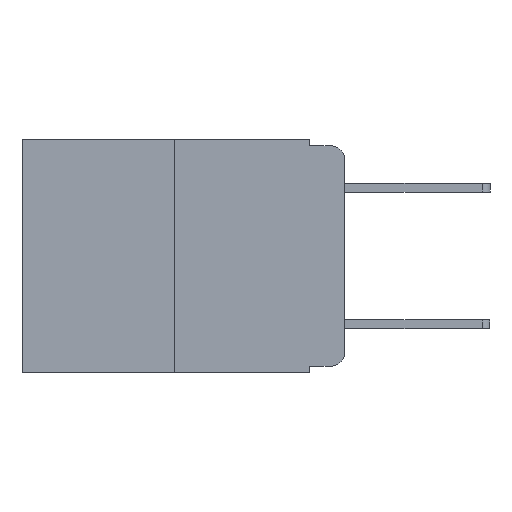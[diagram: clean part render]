
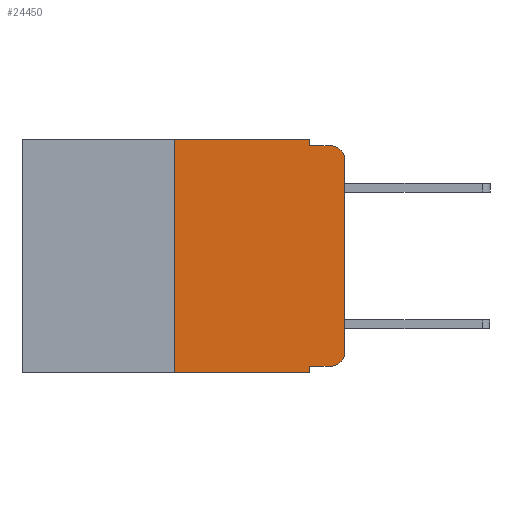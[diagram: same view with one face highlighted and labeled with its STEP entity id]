
A CAD part, left-side view. The second image highlights one B-rep face of the part: STEP entity #24450.
In plain terms, the highlighted planar face has unit normal (-1, 0, 0).
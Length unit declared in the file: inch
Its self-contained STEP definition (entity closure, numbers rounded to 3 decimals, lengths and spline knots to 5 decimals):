
#143 = LINE ( 'NONE', #12916, #20346 ) ;
#436 = CARTESIAN_POINT ( 'NONE',  ( 0., 0.02, -0.01 ) ) ;
#525 = DIRECTION ( 'NONE',  ( 1., 0., 0. ) ) ;
#615 = CARTESIAN_POINT ( 'NONE',  ( 0., 0.051, -0.01 ) ) ;
#1271 = CARTESIAN_POINT ( 'NONE',  ( 0., 0.051, -0.333 ) ) ;
#2166 = VECTOR ( 'NONE', #17414, 39.37008 ) ;
#2287 = EDGE_CURVE ( 'NONE', #21603, #21053, #3094, .T. ) ;
#2307 = VECTOR ( 'NONE', #21862, 39.37008 ) ;
#2392 = CARTESIAN_POINT ( 'NONE',  ( 0., 0.473, -0.343 ) ) ;
#3094 = CIRCLE ( 'NONE', #22832, 0.02 ) ;
#3208 = ORIENTED_EDGE ( 'NONE', *, *, #2287, .T. ) ;
#3269 = CARTESIAN_POINT ( 'NONE',  ( 0., 0., -0.313 ) ) ;
#3487 = CARTESIAN_POINT ( 'NONE',  ( 0., 0.051, 0. ) ) ;
#3617 = EDGE_CURVE ( 'NONE', #11988, #21603, #25023, .T. ) ;
#4017 = CARTESIAN_POINT ( 'NONE',  ( 0., 0.051, 0. ) ) ;
#4315 = VERTEX_POINT ( 'NONE', #22025 ) ;
#4367 = CARTESIAN_POINT ( 'NONE',  ( 0., 0.051, -0.333 ) ) ;
#4509 = DIRECTION ( 'NONE',  ( 0., 0., 1. ) ) ;
#4706 = ORIENTED_EDGE ( 'NONE', *, *, #21992, .F. ) ;
#5257 = VERTEX_POINT ( 'NONE', #15986 ) ;
#5400 = CARTESIAN_POINT ( 'NONE',  ( 0., 0.25, -0.343 ) ) ;
#5429 = DIRECTION ( 'NONE',  ( 0., 0., -1. ) ) ;
#6334 = DIRECTION ( 'NONE',  ( 0., -1., 0. ) ) ;
#6557 = DIRECTION ( 'NONE',  ( 0., -1., 0. ) ) ;
#7359 = LINE ( 'NONE', #4367, #16584 ) ;
#7663 = LINE ( 'NONE', #4017, #12957 ) ;
#7705 = EDGE_CURVE ( 'NONE', #23226, #11988, #23673, .T. ) ;
#7899 = ORIENTED_EDGE ( 'NONE', *, *, #15613, .F. ) ;
#9653 = CARTESIAN_POINT ( 'NONE',  ( 0., 0.25, 0. ) ) ;
#10455 = VECTOR ( 'NONE', #4509, 39.37008 ) ;
#10942 = EDGE_CURVE ( 'NONE', #11424, #5257, #12830, .T. ) ;
#11298 = ORIENTED_EDGE ( 'NONE', *, *, #7705, .T. ) ;
#11424 = VERTEX_POINT ( 'NONE', #5400 ) ;
#11528 = CARTESIAN_POINT ( 'NONE',  ( 0., 0., 0. ) ) ;
#11734 = EDGE_CURVE ( 'NONE', #11986, #23226, #7359, .T. ) ;
#11749 = CARTESIAN_POINT ( 'NONE',  ( 0., 0.02, -0.313 ) ) ;
#11986 = VERTEX_POINT ( 'NONE', #1271 ) ;
#11988 = VERTEX_POINT ( 'NONE', #3269 ) ;
#12208 = AXIS2_PLACEMENT_3D ( 'NONE', #11749, #24976, #13682 ) ;
#12407 = CARTESIAN_POINT ( 'NONE',  ( 0., 0.473, 0. ) ) ;
#12773 = CARTESIAN_POINT ( 'NONE',  ( 0., 0., -0.03 ) ) ;
#12830 = LINE ( 'NONE', #2392, #2307 ) ;
#12916 = CARTESIAN_POINT ( 'NONE',  ( 0., 0.473, 0. ) ) ;
#12957 = VECTOR ( 'NONE', #23291, 39.37008 ) ;
#13430 = EDGE_LOOP ( 'NONE', ( #23753, #3208, #15208, #4706, #21866, #18018, #13774, #7899, #18897, #11298 ) ) ;
#13474 = VECTOR ( 'NONE', #6557, 39.37008 ) ;
#13682 = DIRECTION ( 'NONE',  ( 0., 0., -1. ) ) ;
#13774 = ORIENTED_EDGE ( 'NONE', *, *, #10942, .T. ) ;
#13787 = CARTESIAN_POINT ( 'NONE',  ( 0., 0.051, 0. ) ) ;
#14343 = DIRECTION ( 'NONE',  ( 0., 0., -1. ) ) ;
#15208 = ORIENTED_EDGE ( 'NONE', *, *, #23202, .F. ) ;
#15613 = EDGE_CURVE ( 'NONE', #11986, #5257, #18785, .T. ) ;
#15927 = FACE_OUTER_BOUND ( 'NONE', #13430, .T. ) ;
#15986 = CARTESIAN_POINT ( 'NONE',  ( 0., 0.051, -0.343 ) ) ;
#16584 = VECTOR ( 'NONE', #6334, 39.37008 ) ;
#16934 = EDGE_CURVE ( 'NONE', #11424, #4315, #22257, .T. ) ;
#16974 = VECTOR ( 'NONE', #5429, 39.37008 ) ;
#17348 = EDGE_CURVE ( 'NONE', #4315, #23597, #143, .T. ) ;
#17414 = DIRECTION ( 'NONE',  ( 0., 0., 1. ) ) ;
#17843 = AXIS2_PLACEMENT_3D ( 'NONE', #12407, #525, #14343 ) ;
#18018 = ORIENTED_EDGE ( 'NONE', *, *, #16934, .F. ) ;
#18288 = CARTESIAN_POINT ( 'NONE',  ( 0., 0.02, -0.333 ) ) ;
#18625 = LINE ( 'NONE', #615, #13474 ) ;
#18636 = VERTEX_POINT ( 'NONE', #21741 ) ;
#18754 = DIRECTION ( 'NONE',  ( 0., -1., 0. ) ) ;
#18785 = LINE ( 'NONE', #3487, #16974 ) ;
#18897 = ORIENTED_EDGE ( 'NONE', *, *, #11734, .T. ) ;
#19837 = DIRECTION ( 'NONE',  ( -1., 0., 0. ) ) ;
#19894 = CARTESIAN_POINT ( 'NONE',  ( 0., 0.02, -0.03 ) ) ;
#20028 = PLANE ( 'NONE',  #17843 ) ;
#20346 = VECTOR ( 'NONE', #18754, 39.37008 ) ;
#21053 = VERTEX_POINT ( 'NONE', #436 ) ;
#21603 = VERTEX_POINT ( 'NONE', #12773 ) ;
#21741 = CARTESIAN_POINT ( 'NONE',  ( 0., 0.051, -0.01 ) ) ;
#21763 = DIRECTION ( 'NONE',  ( 0., 0., -1. ) ) ;
#21862 = DIRECTION ( 'NONE',  ( 0., -1., 0. ) ) ;
#21866 = ORIENTED_EDGE ( 'NONE', *, *, #17348, .F. ) ;
#21992 = EDGE_CURVE ( 'NONE', #23597, #18636, #7663, .T. ) ;
#22025 = CARTESIAN_POINT ( 'NONE',  ( 0., 0.25, 0. ) ) ;
#22257 = LINE ( 'NONE', #9653, #2166 ) ;
#22832 = AXIS2_PLACEMENT_3D ( 'NONE', #19894, #19837, #21763 ) ;
#23202 = EDGE_CURVE ( 'NONE', #18636, #21053, #18625, .T. ) ;
#23226 = VERTEX_POINT ( 'NONE', #18288 ) ;
#23291 = DIRECTION ( 'NONE',  ( 0., 0., -1. ) ) ;
#23597 = VERTEX_POINT ( 'NONE', #13787 ) ;
#23673 = CIRCLE ( 'NONE', #12208, 0.02 ) ;
#23753 = ORIENTED_EDGE ( 'NONE', *, *, #3617, .T. ) ;
#24450 = ADVANCED_FACE ( 'NONE', ( #15927 ), #20028, .F. ) ;
#24976 = DIRECTION ( 'NONE',  ( -1., 0., 0. ) ) ;
#25023 = LINE ( 'NONE', #11528, #10455 ) ;
